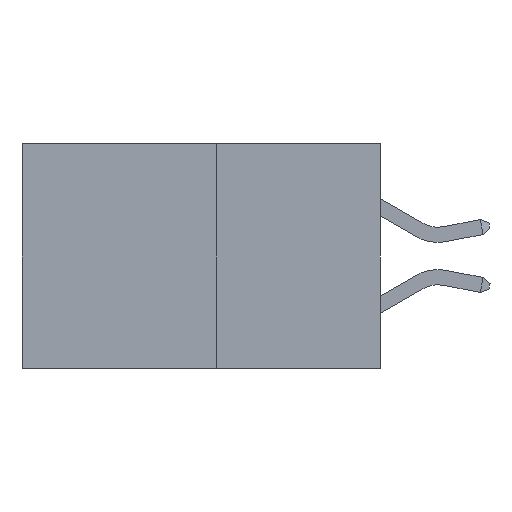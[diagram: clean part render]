
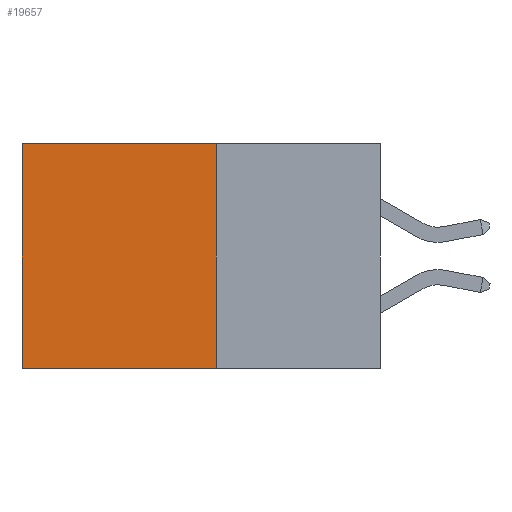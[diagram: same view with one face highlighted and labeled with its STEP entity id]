
A CAD part, left-side view. The second image highlights one B-rep face of the part: STEP entity #19657.
In plain terms, the highlighted planar face has unit normal (-1, 0, 0).
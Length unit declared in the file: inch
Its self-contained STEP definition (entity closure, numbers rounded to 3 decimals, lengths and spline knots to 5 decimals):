
#1907 = DIRECTION ( 'NONE',  ( 1., 0., 0. ) ) ;
#2743 = AXIS2_PLACEMENT_3D ( 'NONE', #12047, #1907, #13583 ) ;
#2750 = CARTESIAN_POINT ( 'NONE',  ( 0.277, 0.27, 0. ) ) ;
#3410 = DIRECTION ( 'NONE',  ( 0., 1., 0. ) ) ;
#3470 = VECTOR ( 'NONE', #3988, 39.37008 ) ;
#3702 = CARTESIAN_POINT ( 'NONE',  ( 0.277, 0.59, 0. ) ) ;
#3951 = EDGE_CURVE ( 'NONE', #7546, #11192, #11913, .T. ) ;
#3988 = DIRECTION ( 'NONE',  ( 0., 0., -1. ) ) ;
#4025 = VERTEX_POINT ( 'NONE', #3702 ) ;
#4386 = FACE_OUTER_BOUND ( 'NONE', #16356, .T. ) ;
#4616 = CARTESIAN_POINT ( 'NONE',  ( 0.277, 0.27, -0.37 ) ) ;
#5250 = CARTESIAN_POINT ( 'NONE',  ( 0.277, 0.59, -0.37 ) ) ;
#5317 = PLANE ( 'NONE',  #2743 ) ;
#6086 = DIRECTION ( 'NONE',  ( 0., 1., 0. ) ) ;
#7142 = VERTEX_POINT ( 'NONE', #5250 ) ;
#7546 = VERTEX_POINT ( 'NONE', #2750 ) ;
#8812 = CARTESIAN_POINT ( 'NONE',  ( 0.277, 0.59, -0.37 ) ) ;
#10103 = VECTOR ( 'NONE', #19709, 39.37008 ) ;
#11083 = CARTESIAN_POINT ( 'NONE',  ( 0.277, 0.27, 0. ) ) ;
#11121 = LINE ( 'NONE', #8812, #10103 ) ;
#11192 = VERTEX_POINT ( 'NONE', #4616 ) ;
#11913 = LINE ( 'NONE', #12084, #3470 ) ;
#12047 = CARTESIAN_POINT ( 'NONE',  ( 0.277, 0.27, -0.37 ) ) ;
#12084 = CARTESIAN_POINT ( 'NONE',  ( 0.277, 0.27, -0.37 ) ) ;
#12206 = EDGE_CURVE ( 'NONE', #4025, #7142, #11121, .T. ) ;
#12778 = EDGE_CURVE ( 'NONE', #11192, #7142, #16771, .T. ) ;
#13372 = CARTESIAN_POINT ( 'NONE',  ( 0.277, 0.27, -0.37 ) ) ;
#13583 = DIRECTION ( 'NONE',  ( 0., 0., -1. ) ) ;
#14804 = VECTOR ( 'NONE', #6086, 39.37008 ) ;
#16049 = EDGE_CURVE ( 'NONE', #7546, #4025, #18801, .T. ) ;
#16292 = VECTOR ( 'NONE', #3410, 39.37008 ) ;
#16356 = EDGE_LOOP ( 'NONE', ( #20311, #20328, #19889, #17512 ) ) ;
#16771 = LINE ( 'NONE', #13372, #16292 ) ;
#17512 = ORIENTED_EDGE ( 'NONE', *, *, #16049, .T. ) ;
#18801 = LINE ( 'NONE', #11083, #14804 ) ;
#19657 = ADVANCED_FACE ( 'NONE', ( #4386 ), #5317, .F. ) ;
#19709 = DIRECTION ( 'NONE',  ( 0., 0., -1. ) ) ;
#19889 = ORIENTED_EDGE ( 'NONE', *, *, #3951, .F. ) ;
#20311 = ORIENTED_EDGE ( 'NONE', *, *, #12206, .T. ) ;
#20328 = ORIENTED_EDGE ( 'NONE', *, *, #12778, .F. ) ;
